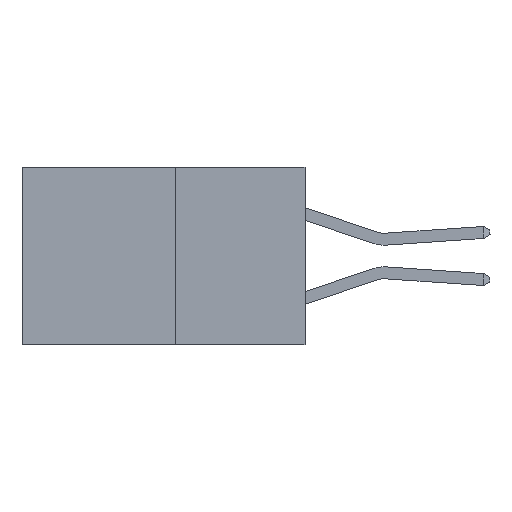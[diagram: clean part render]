
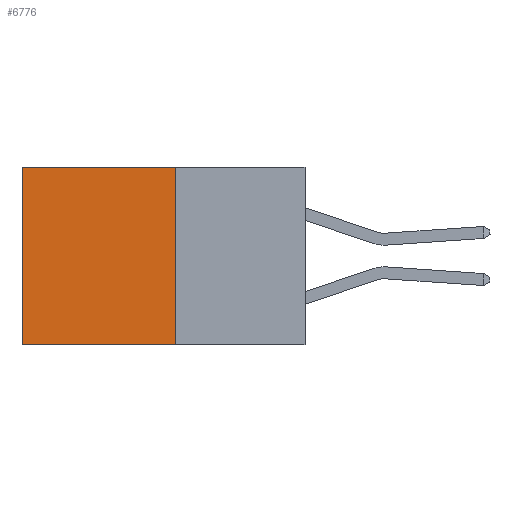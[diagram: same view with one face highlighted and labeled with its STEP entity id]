
A CAD part, left-side view. The second image highlights one B-rep face of the part: STEP entity #6776.
In plain terms, the highlighted planar face has unit normal (-1, 0, 0).
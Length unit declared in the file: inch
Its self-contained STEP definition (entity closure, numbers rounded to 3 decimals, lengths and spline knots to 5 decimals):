
#729 = LINE ( 'NONE', #11502, #28105 ) ;
#3099 = LINE ( 'NONE', #5643, #25976 ) ;
#4539 = EDGE_CURVE ( 'NONE', #24823, #26486, #729, .T. ) ;
#5601 = CARTESIAN_POINT ( 'NONE',  ( 0.277, 0.27, 0. ) ) ;
#5643 = CARTESIAN_POINT ( 'NONE',  ( 0.277, 0.27, -0.37 ) ) ;
#6310 = VECTOR ( 'NONE', #20991, 39.37008 ) ;
#6776 = ADVANCED_FACE ( 'NONE', ( #27937 ), #15278, .F. ) ;
#9979 = CARTESIAN_POINT ( 'NONE',  ( 0.277, 0.59, -0.37 ) ) ;
#10721 = CARTESIAN_POINT ( 'NONE',  ( 0.277, 0.59, -0.37 ) ) ;
#11502 = CARTESIAN_POINT ( 'NONE',  ( 0.277, 0.27, -0.37 ) ) ;
#11699 = CARTESIAN_POINT ( 'NONE',  ( 0.277, 0.27, -0.37 ) ) ;
#13202 = VECTOR ( 'NONE', #21090, 39.37008 ) ;
#13780 = CARTESIAN_POINT ( 'NONE',  ( 0.277, 0.59, 0. ) ) ;
#14638 = DIRECTION ( 'NONE',  ( 0., 0., -1. ) ) ;
#15183 = DIRECTION ( 'NONE',  ( 0., 0., -1. ) ) ;
#15204 = DIRECTION ( 'NONE',  ( 1., 0., 0. ) ) ;
#15278 = PLANE ( 'NONE',  #21583 ) ;
#15463 = CARTESIAN_POINT ( 'NONE',  ( 0.277, 0.27, -0.37 ) ) ;
#16427 = VERTEX_POINT ( 'NONE', #10721 ) ;
#18537 = EDGE_CURVE ( 'NONE', #26486, #16427, #3099, .T. ) ;
#19498 = CARTESIAN_POINT ( 'NONE',  ( 0.277, 0.27, 0. ) ) ;
#20319 = ORIENTED_EDGE ( 'NONE', *, *, #4539, .F. ) ;
#20991 = DIRECTION ( 'NONE',  ( 0., 0., -1. ) ) ;
#21090 = DIRECTION ( 'NONE',  ( 0., 1., 0. ) ) ;
#21583 = AXIS2_PLACEMENT_3D ( 'NONE', #15463, #15204, #15183 ) ;
#22346 = EDGE_CURVE ( 'NONE', #23717, #16427, #23959, .T. ) ;
#23717 = VERTEX_POINT ( 'NONE', #13780 ) ;
#23959 = LINE ( 'NONE', #9979, #6310 ) ;
#24092 = ORIENTED_EDGE ( 'NONE', *, *, #22346, .T. ) ;
#24823 = VERTEX_POINT ( 'NONE', #19498 ) ;
#25499 = ORIENTED_EDGE ( 'NONE', *, *, #27398, .T. ) ;
#25976 = VECTOR ( 'NONE', #27680, 39.37008 ) ;
#26486 = VERTEX_POINT ( 'NONE', #11699 ) ;
#26784 = EDGE_LOOP ( 'NONE', ( #24092, #28262, #20319, #25499 ) ) ;
#27398 = EDGE_CURVE ( 'NONE', #24823, #23717, #28014, .T. ) ;
#27680 = DIRECTION ( 'NONE',  ( 0., 1., 0. ) ) ;
#27937 = FACE_OUTER_BOUND ( 'NONE', #26784, .T. ) ;
#28014 = LINE ( 'NONE', #5601, #13202 ) ;
#28105 = VECTOR ( 'NONE', #14638, 39.37008 ) ;
#28262 = ORIENTED_EDGE ( 'NONE', *, *, #18537, .F. ) ;
